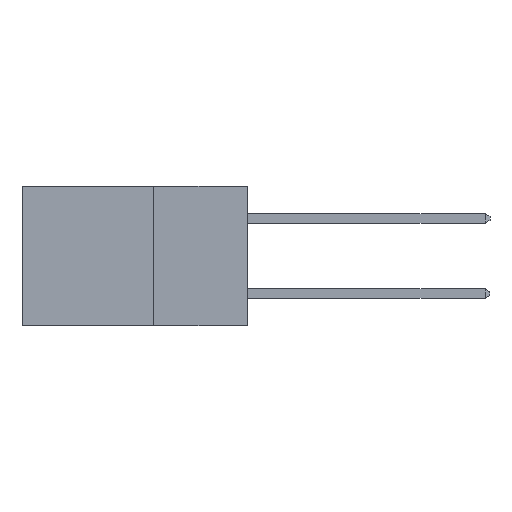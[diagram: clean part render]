
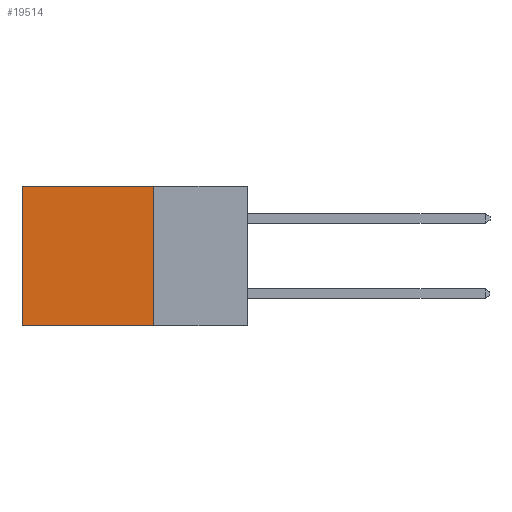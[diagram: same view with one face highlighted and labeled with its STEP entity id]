
A CAD part, left-side view. The second image highlights one B-rep face of the part: STEP entity #19514.
In plain terms, the highlighted planar face has unit normal (-1, 0, 0).
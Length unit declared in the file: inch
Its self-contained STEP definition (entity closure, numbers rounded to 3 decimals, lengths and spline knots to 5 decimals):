
#693 = FACE_OUTER_BOUND ( 'NONE', #2475, .T. ) ;
#696 = LINE ( 'NONE', #15953, #4462 ) ;
#1008 = DIRECTION ( 'NONE',  ( 0., 0., -1. ) ) ;
#1115 = ORIENTED_EDGE ( 'NONE', *, *, #7464, .F. ) ;
#2475 = EDGE_LOOP ( 'NONE', ( #18465, #14138, #1115, #13308 ) ) ;
#2694 = VERTEX_POINT ( 'NONE', #12950 ) ;
#3183 = VECTOR ( 'NONE', #9472, 39.37008 ) ;
#4326 = VECTOR ( 'NONE', #14485, 39.37008 ) ;
#4462 = VECTOR ( 'NONE', #4648, 39.37008 ) ;
#4648 = DIRECTION ( 'NONE',  ( 0., 0., -1. ) ) ;
#5049 = EDGE_CURVE ( 'NONE', #5344, #18620, #17207, .T. ) ;
#5344 = VERTEX_POINT ( 'NONE', #13706 ) ;
#6447 = PLANE ( 'NONE',  #12347 ) ;
#7464 = EDGE_CURVE ( 'NONE', #5344, #2694, #696, .T. ) ;
#8656 = EDGE_CURVE ( 'NONE', #2694, #9049, #16575, .T. ) ;
#9049 = VERTEX_POINT ( 'NONE', #13531 ) ;
#9472 = DIRECTION ( 'NONE',  ( 0., 1., 0. ) ) ;
#9693 = DIRECTION ( 'NONE',  ( 0., 0., -1. ) ) ;
#12347 = AXIS2_PLACEMENT_3D ( 'NONE', #17756, #19364, #9693 ) ;
#12876 = CARTESIAN_POINT ( 'NONE',  ( 0.298, 0.25, 0. ) ) ;
#12950 = CARTESIAN_POINT ( 'NONE',  ( 0.298, 0.25, -0.37 ) ) ;
#13308 = ORIENTED_EDGE ( 'NONE', *, *, #5049, .T. ) ;
#13531 = CARTESIAN_POINT ( 'NONE',  ( 0.298, 0.6, -0.37 ) ) ;
#13595 = VECTOR ( 'NONE', #1008, 39.37008 ) ;
#13706 = CARTESIAN_POINT ( 'NONE',  ( 0.298, 0.25, 0. ) ) ;
#14095 = LINE ( 'NONE', #20283, #13595 ) ;
#14138 = ORIENTED_EDGE ( 'NONE', *, *, #8656, .F. ) ;
#14485 = DIRECTION ( 'NONE',  ( 0., 1., 0. ) ) ;
#14915 = EDGE_CURVE ( 'NONE', #18620, #9049, #14095, .T. ) ;
#15953 = CARTESIAN_POINT ( 'NONE',  ( 0.298, 0.25, 0. ) ) ;
#16575 = LINE ( 'NONE', #17514, #3183 ) ;
#17207 = LINE ( 'NONE', #12876, #4326 ) ;
#17514 = CARTESIAN_POINT ( 'NONE',  ( 0.298, 0.25, -0.37 ) ) ;
#17756 = CARTESIAN_POINT ( 'NONE',  ( 0.298, 0.25, 0. ) ) ;
#18465 = ORIENTED_EDGE ( 'NONE', *, *, #14915, .T. ) ;
#18620 = VERTEX_POINT ( 'NONE', #18760 ) ;
#18760 = CARTESIAN_POINT ( 'NONE',  ( 0.298, 0.6, 0. ) ) ;
#19364 = DIRECTION ( 'NONE',  ( 1., 0., 0. ) ) ;
#19514 = ADVANCED_FACE ( 'NONE', ( #693 ), #6447, .F. ) ;
#20283 = CARTESIAN_POINT ( 'NONE',  ( 0.298, 0.6, 0. ) ) ;
